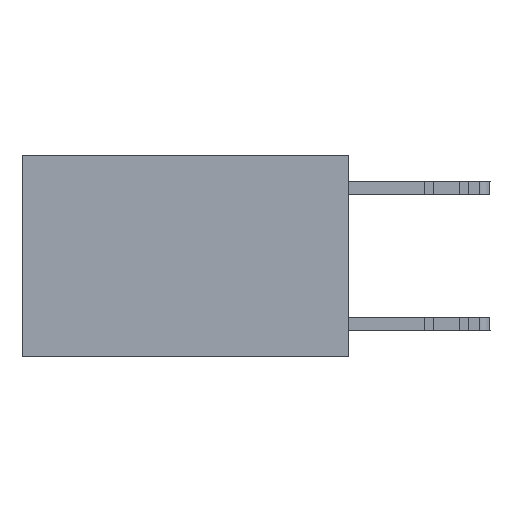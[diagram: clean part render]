
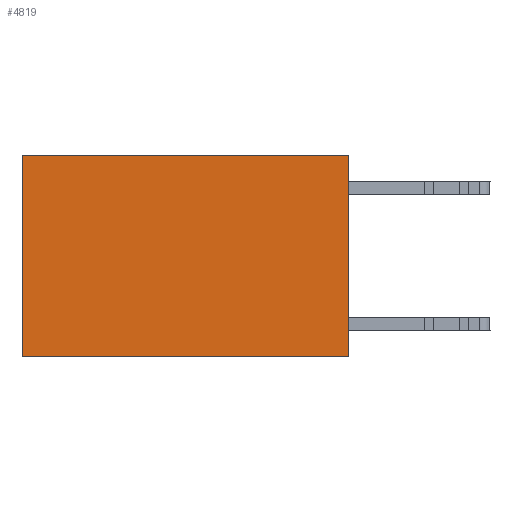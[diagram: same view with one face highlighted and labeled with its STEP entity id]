
A CAD part, left-side view. The second image highlights one B-rep face of the part: STEP entity #4819.
In plain terms, the highlighted planar face has unit normal (-1, 0, 0).
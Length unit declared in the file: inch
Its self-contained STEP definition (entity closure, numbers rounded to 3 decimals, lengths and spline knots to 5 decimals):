
#192 = CARTESIAN_POINT ( 'NONE',  ( 0.2625, 0., 0. ) ) ;
#1239 = CARTESIAN_POINT ( 'NONE',  ( 0.2625, 0., -0.37 ) ) ;
#1940 = VERTEX_POINT ( 'NONE', #1239 ) ;
#2395 = VERTEX_POINT ( 'NONE', #192 ) ;
#2824 = LINE ( 'NONE', #5010, #13168 ) ;
#3061 = DIRECTION ( 'NONE',  ( 0., 0., -1. ) ) ;
#3377 = DIRECTION ( 'NONE',  ( 0., 1., 0. ) ) ;
#4819 = ADVANCED_FACE ( 'NONE', ( #24384 ), #24847, .F. ) ;
#5010 = CARTESIAN_POINT ( 'NONE',  ( 0.2625, 0., 0. ) ) ;
#5748 = LINE ( 'NONE', #15266, #10035 ) ;
#5889 = VECTOR ( 'NONE', #3377, 39.37008 ) ;
#7661 = EDGE_CURVE ( 'NONE', #17271, #11520, #5748, .T. ) ;
#9017 = ORIENTED_EDGE ( 'NONE', *, *, #7661, .T. ) ;
#10035 = VECTOR ( 'NONE', #12908, 39.37008 ) ;
#10383 = ORIENTED_EDGE ( 'NONE', *, *, #23376, .F. ) ;
#11384 = CARTESIAN_POINT ( 'NONE',  ( 0.2625, 0.6, 0. ) ) ;
#11478 = ORIENTED_EDGE ( 'NONE', *, *, #15645, .T. ) ;
#11520 = VERTEX_POINT ( 'NONE', #25606 ) ;
#12908 = DIRECTION ( 'NONE',  ( 0., 0., -1. ) ) ;
#13168 = VECTOR ( 'NONE', #24444, 39.37008 ) ;
#13488 = LINE ( 'NONE', #27821, #5889 ) ;
#15266 = CARTESIAN_POINT ( 'NONE',  ( 0.2625, 0.6, 0. ) ) ;
#15376 = CARTESIAN_POINT ( 'NONE',  ( 0.2625, 0., 0. ) ) ;
#15645 = EDGE_CURVE ( 'NONE', #2395, #17271, #2824, .T. ) ;
#17271 = VERTEX_POINT ( 'NONE', #11384 ) ;
#19849 = AXIS2_PLACEMENT_3D ( 'NONE', #15376, #29525, #3061 ) ;
#22722 = LINE ( 'NONE', #25369, #29592 ) ;
#23376 = EDGE_CURVE ( 'NONE', #1940, #11520, #13488, .T. ) ;
#24384 = FACE_OUTER_BOUND ( 'NONE', #27851, .T. ) ;
#24444 = DIRECTION ( 'NONE',  ( 0., 1., 0. ) ) ;
#24847 = PLANE ( 'NONE',  #19849 ) ;
#25219 = DIRECTION ( 'NONE',  ( 0., 0., -1. ) ) ;
#25369 = CARTESIAN_POINT ( 'NONE',  ( 0.2625, 0., 0. ) ) ;
#25606 = CARTESIAN_POINT ( 'NONE',  ( 0.2625, 0.6, -0.37 ) ) ;
#27821 = CARTESIAN_POINT ( 'NONE',  ( 0.2625, 0., -0.37 ) ) ;
#27851 = EDGE_LOOP ( 'NONE', ( #9017, #10383, #28725, #11478 ) ) ;
#28725 = ORIENTED_EDGE ( 'NONE', *, *, #29311, .F. ) ;
#29311 = EDGE_CURVE ( 'NONE', #2395, #1940, #22722, .T. ) ;
#29525 = DIRECTION ( 'NONE',  ( 1., 0., 0. ) ) ;
#29592 = VECTOR ( 'NONE', #25219, 39.37008 ) ;
